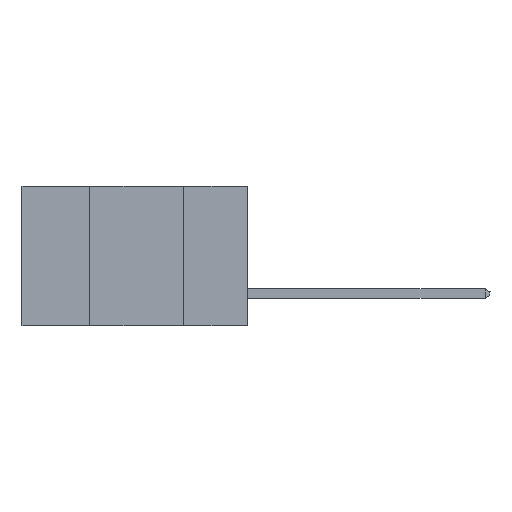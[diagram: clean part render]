
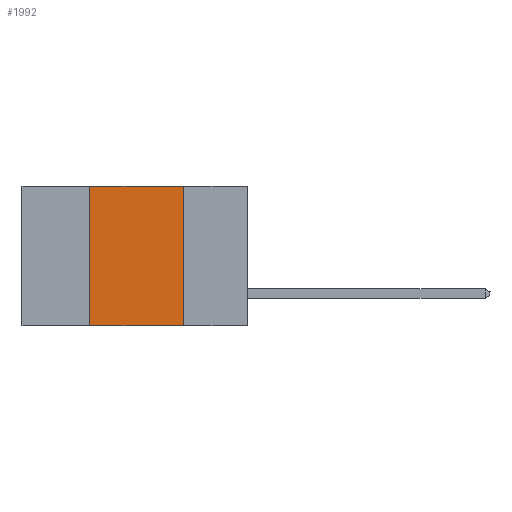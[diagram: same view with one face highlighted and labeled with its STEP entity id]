
A CAD part, left-side view. The second image highlights one B-rep face of the part: STEP entity #1992.
In plain terms, the highlighted planar face has unit normal (-1, 0, 0).
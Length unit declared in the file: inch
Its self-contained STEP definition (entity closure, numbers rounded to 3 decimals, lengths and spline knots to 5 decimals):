
#620 = VECTOR ( 'NONE', #9170, 39.37008 ) ;
#1073 = VERTEX_POINT ( 'NONE', #20504 ) ;
#1363 = DIRECTION ( 'NONE',  ( 1., 0., 0. ) ) ;
#1992 = ADVANCED_FACE ( 'NONE', ( #18438 ), #3058, .F. ) ;
#3058 = PLANE ( 'NONE',  #11086 ) ;
#3579 = VECTOR ( 'NONE', #16175, 39.37008 ) ;
#3984 = VERTEX_POINT ( 'NONE', #14640 ) ;
#4080 = LINE ( 'NONE', #5876, #7908 ) ;
#4480 = EDGE_LOOP ( 'NONE', ( #15553, #21393, #16564, #7195 ) ) ;
#5213 = DIRECTION ( 'NONE',  ( 0., 0., -1. ) ) ;
#5428 = VERTEX_POINT ( 'NONE', #22199 ) ;
#5818 = LINE ( 'NONE', #5916, #620 ) ;
#5876 = CARTESIAN_POINT ( 'NONE',  ( 0., 0.6, -0.37 ) ) ;
#5916 = CARTESIAN_POINT ( 'NONE',  ( 0., 0.6, 0. ) ) ;
#6206 = VERTEX_POINT ( 'NONE', #14380 ) ;
#6729 = VECTOR ( 'NONE', #5213, 39.37008 ) ;
#7195 = ORIENTED_EDGE ( 'NONE', *, *, #13713, .T. ) ;
#7416 = EDGE_CURVE ( 'NONE', #3984, #6206, #7750, .T. ) ;
#7750 = LINE ( 'NONE', #9345, #3579 ) ;
#7908 = VECTOR ( 'NONE', #20225, 39.37008 ) ;
#9170 = DIRECTION ( 'NONE',  ( 0., -1., 0. ) ) ;
#9345 = CARTESIAN_POINT ( 'NONE',  ( 0., 0.42, -0.37 ) ) ;
#10415 = EDGE_CURVE ( 'NONE', #1073, #5428, #13292, .T. ) ;
#11086 = AXIS2_PLACEMENT_3D ( 'NONE', #16724, #1363, #19804 ) ;
#13292 = LINE ( 'NONE', #15288, #6729 ) ;
#13713 = EDGE_CURVE ( 'NONE', #3984, #5428, #4080, .T. ) ;
#14380 = CARTESIAN_POINT ( 'NONE',  ( 0., 0.42, 0. ) ) ;
#14640 = CARTESIAN_POINT ( 'NONE',  ( 0., 0.42, -0.37 ) ) ;
#15288 = CARTESIAN_POINT ( 'NONE',  ( 0., 0.17, -0.37 ) ) ;
#15553 = ORIENTED_EDGE ( 'NONE', *, *, #10415, .F. ) ;
#16175 = DIRECTION ( 'NONE',  ( 0., 0., 1. ) ) ;
#16323 = EDGE_CURVE ( 'NONE', #6206, #1073, #5818, .T. ) ;
#16564 = ORIENTED_EDGE ( 'NONE', *, *, #7416, .F. ) ;
#16724 = CARTESIAN_POINT ( 'NONE',  ( 0., 0.6, 0. ) ) ;
#18438 = FACE_OUTER_BOUND ( 'NONE', #4480, .T. ) ;
#19804 = DIRECTION ( 'NONE',  ( 0., 0., -1. ) ) ;
#20225 = DIRECTION ( 'NONE',  ( 0., -1., 0. ) ) ;
#20504 = CARTESIAN_POINT ( 'NONE',  ( 0., 0.17, 0. ) ) ;
#21393 = ORIENTED_EDGE ( 'NONE', *, *, #16323, .F. ) ;
#22199 = CARTESIAN_POINT ( 'NONE',  ( 0., 0.17, -0.37 ) ) ;
